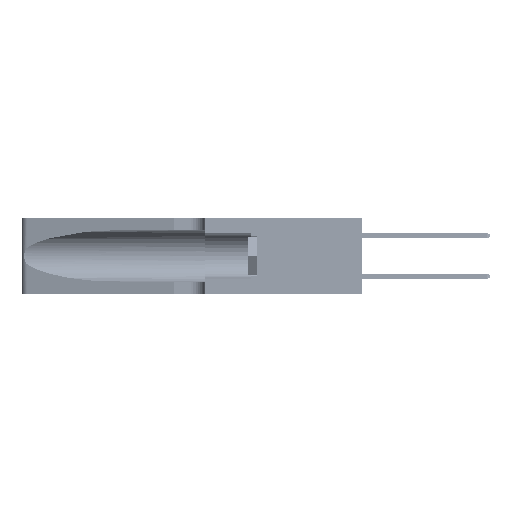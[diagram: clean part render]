
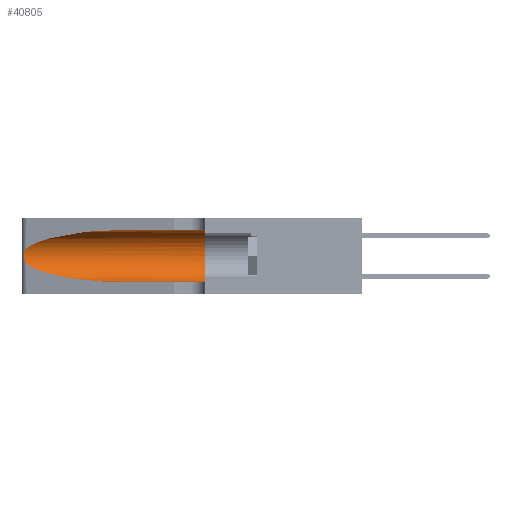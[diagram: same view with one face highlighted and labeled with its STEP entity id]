
A CAD part, left-side view. The second image highlights one B-rep face of the part: STEP entity #40805.
In plain terms, the highlighted cylindrical face has radius 3.308 mm (diameter 6.617 mm), a partial arc.
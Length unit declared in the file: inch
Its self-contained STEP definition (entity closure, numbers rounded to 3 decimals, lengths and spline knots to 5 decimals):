
#944 = EDGE_CURVE ( 'NONE', #6087, #50796, #41452, .T. ) ;
#1421 = CARTESIAN_POINT ( 'NONE',  ( 0.25487, 1.22718, 0.22369 ) ) ;
#3061 = DIRECTION ( 'NONE',  ( 0., -1., 0. ) ) ;
#3164 = CARTESIAN_POINT ( 'NONE',  ( 0.26017, 1.23833, 0.17102 ) ) ;
#3268 = ORIENTED_EDGE ( 'NONE', *, *, #46755, .T. ) ;
#3744 = VERTEX_POINT ( 'NONE', #12355 ) ;
#3941 = CARTESIAN_POINT ( 'NONE',  ( 0.1305, 0.72297, 0.05475 ) ) ;
#5886 = ORIENTED_EDGE ( 'NONE', *, *, #34191, .T. ) ;
#6087 = VERTEX_POINT ( 'NONE', #18810 ) ;
#7437 = CARTESIAN_POINT ( 'NONE',  ( 0.25789, 1.23486, 0.15765 ) ) ;
#8527 = CARTESIAN_POINT ( 'NONE',  ( 0.1305, 0.72297, 0.05475 ) ) ;
#8757 = EDGE_CURVE ( 'NONE', #24633, #31494, #41089, .T. ) ;
#9871 = ORIENTED_EDGE ( 'NONE', *, *, #944, .T. ) ;
#11133 = CYLINDRICAL_SURFACE ( 'NONE', #44192, 0.13025 ) ;
#11691 = CARTESIAN_POINT ( 'NONE',  ( 0.25555, 1.22993, 0.14849 ) ) ;
#12355 = CARTESIAN_POINT ( 'NONE',  ( 0.1305, 0.72297, 0.31525 ) ) ;
#14415 = EDGE_CURVE ( 'NONE', #18803, #31494, #33669, .T. ) ;
#14484 = DIRECTION ( 'NONE',  ( 0., 1., 0. ) ) ;
#16391 = CARTESIAN_POINT ( 'NONE',  ( 0.25487, 1.22718, 0.22369 ) ) ;
#16529 = CARTESIAN_POINT ( 'NONE',  ( 0.25487, 1.22718, 0.14631 ) ) ;
#17696 =( BOUNDED_CURVE ( )  B_SPLINE_CURVE ( 3, ( #16529, #33474, #29374, #3941 ),
 .UNSPECIFIED., .F., .F. ) 
 B_SPLINE_CURVE_WITH_KNOTS ( ( 4, 4 ),
 ( 3.44316, 4.71239 ),
 .UNSPECIFIED. ) 
 CURVE ( )  GEOMETRIC_REPRESENTATION_ITEM ( )  RATIONAL_B_SPLINE_CURVE ( ( 1., 0.87, 0.87, 1. ) ) 
 REPRESENTATION_ITEM ( '' )  );
#18803 = VERTEX_POINT ( 'NONE', #8527 ) ;
#18810 = CARTESIAN_POINT ( 'NONE',  ( 0.25487, 1.22718, 0.22369 ) ) ;
#19233 = CARTESIAN_POINT ( 'NONE',  ( 0.1305, 1.61858, 0.31525 ) ) ;
#22377 = VECTOR ( 'NONE', #37004, 39.37008 ) ;
#23719 = CARTESIAN_POINT ( 'NONE',  ( 0.25487, 1.22718, 0.14631 ) ) ;
#23784 = FACE_OUTER_BOUND ( 'NONE', #28437, .T. ) ;
#24243 = CARTESIAN_POINT ( 'NONE',  ( 0.1305, 1.61858, 0.05475 ) ) ;
#24633 = VERTEX_POINT ( 'NONE', #26591 ) ;
#25056 = ORIENTED_EDGE ( 'NONE', *, *, #8757, .F. ) ;
#26591 = CARTESIAN_POINT ( 'NONE',  ( 0.1305, 0.35, 0.31525 ) ) ;
#26876 = CARTESIAN_POINT ( 'NONE',  ( 0.25555, 1.22994, 0.2215 ) ) ;
#27770 = DIRECTION ( 'NONE',  ( 0., -1., 0. ) ) ;
#28437 = EDGE_LOOP ( 'NONE', ( #3268, #9871, #5886, #38956, #25056, #53996 ) ) ;
#28609 = CARTESIAN_POINT ( 'NONE',  ( 0.26075, 1.23896, 0.178 ) ) ;
#28958 = CARTESIAN_POINT ( 'NONE',  ( 0.25787, 1.23484, 0.2124 ) ) ;
#29374 = CARTESIAN_POINT ( 'NONE',  ( 0.18966, 0.96281, 0.05475 ) ) ;
#30862 = EDGE_CURVE ( 'NONE', #3744, #24633, #47427, .T. ) ;
#31494 = VERTEX_POINT ( 'NONE', #52696 ) ;
#32801 = DIRECTION ( 'NONE',  ( 0., 0., -1. ) ) ;
#32897 = CARTESIAN_POINT ( 'NONE',  ( 0.25856, 1.23593, 0.16098 ) ) ;
#33347 = CARTESIAN_POINT ( 'NONE',  ( 0.1305, 0.72297, 0.31525 ) ) ;
#33448 = CARTESIAN_POINT ( 'NONE',  ( 0.26018, 1.23835, 0.19895 ) ) ;
#33474 = CARTESIAN_POINT ( 'NONE',  ( 0.2373, 1.15595, 0.08982 ) ) ;
#33572 = CARTESIAN_POINT ( 'NONE',  ( 0.25639, 1.23184, 0.21858 ) ) ;
#33669 = LINE ( 'NONE', #24243, #22377 ) ;
#34191 = EDGE_CURVE ( 'NONE', #50796, #18803, #17696, .T. ) ;
#37004 = DIRECTION ( 'NONE',  ( 0., -1., 0. ) ) ;
#37109 = CARTESIAN_POINT ( 'NONE',  ( 0.25639, 1.23186, 0.15144 ) ) ;
#37197 = AXIS2_PLACEMENT_3D ( 'NONE', #39899, #14484, #44133 ) ;
#37570 = VECTOR ( 'NONE', #27770, 39.37008 ) ;
#38956 = ORIENTED_EDGE ( 'NONE', *, *, #14415, .T. ) ;
#39899 = CARTESIAN_POINT ( 'NONE',  ( 0.1305, 0.35, 0.185 ) ) ;
#40805 = ADVANCED_FACE ( 'NONE', ( #23784 ), #11133, .F. ) ;
#41027 = CARTESIAN_POINT ( 'NONE',  ( 0.25854, 1.2359, 0.20912 ) ) ;
#41060 = CARTESIAN_POINT ( 'NONE',  ( 0.1305, 1.61858, 0.185 ) ) ;
#41089 = CIRCLE ( 'NONE', #37197, 0.13025 ) ;
#41318 = CARTESIAN_POINT ( 'NONE',  ( 0.25487, 1.22718, 0.14631 ) ) ;
#41452 = B_SPLINE_CURVE_WITH_KNOTS ( 'NONE', 3,
 ( #1421, #26876, #33572, #28958, #41027, #33448, #53771, #28609, #3164, #32897, #7437, #37109, #11691, #41318 ),
 .UNSPECIFIED., .F., .F.,
 ( 4, 2, 2, 2, 2, 2, 4 ),
 ( 0., 0.00027, 0.00053, 0.00107, 0.0016, 0.00187, 0.00214 ),
 .UNSPECIFIED. ) ;
#41785 = CARTESIAN_POINT ( 'NONE',  ( 0.2373, 1.15595, 0.28018 ) ) ;
#43145 =( BOUNDED_CURVE ( )  B_SPLINE_CURVE ( 3, ( #33347, #54226, #41785, #16391 ),
 .UNSPECIFIED., .F., .T. ) 
 B_SPLINE_CURVE_WITH_KNOTS ( ( 4, 4 ),
 ( 1.5708, 2.84003 ),
 .UNSPECIFIED. ) 
 CURVE ( )  GEOMETRIC_REPRESENTATION_ITEM ( )  RATIONAL_B_SPLINE_CURVE ( ( 1., 0.87, 0.87, 1. ) ) 
 REPRESENTATION_ITEM ( '' )  );
#44133 = DIRECTION ( 'NONE',  ( 0., 0., 1. ) ) ;
#44192 = AXIS2_PLACEMENT_3D ( 'NONE', #41060, #3061, #32801 ) ;
#46755 = EDGE_CURVE ( 'NONE', #3744, #6087, #43145, .T. ) ;
#47427 = LINE ( 'NONE', #19233, #37570 ) ;
#50796 = VERTEX_POINT ( 'NONE', #23719 ) ;
#52696 = CARTESIAN_POINT ( 'NONE',  ( 0.1305, 0.35, 0.05475 ) ) ;
#53771 = CARTESIAN_POINT ( 'NONE',  ( 0.26075, 1.23896, 0.19203 ) ) ;
#53996 = ORIENTED_EDGE ( 'NONE', *, *, #30862, .F. ) ;
#54226 = CARTESIAN_POINT ( 'NONE',  ( 0.18966, 0.96281, 0.31525 ) ) ;
